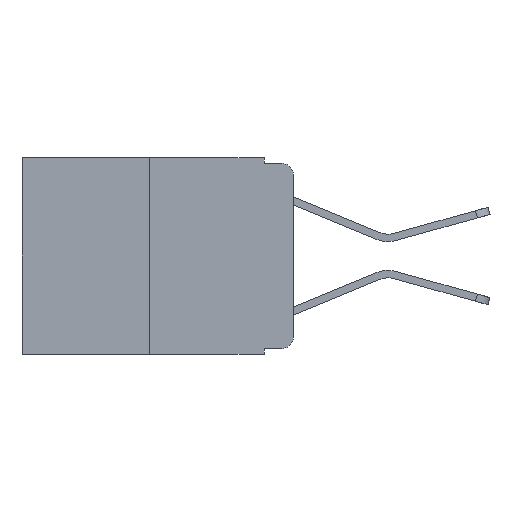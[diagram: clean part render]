
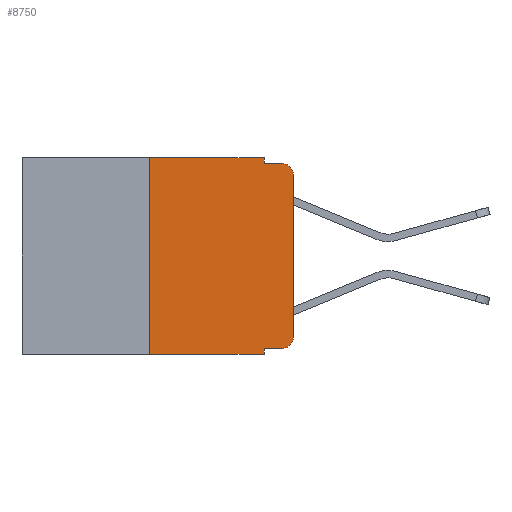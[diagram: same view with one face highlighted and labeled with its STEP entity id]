
A CAD part, left-side view. The second image highlights one B-rep face of the part: STEP entity #8750.
In plain terms, the highlighted planar face has unit normal (-1, 0, 0).
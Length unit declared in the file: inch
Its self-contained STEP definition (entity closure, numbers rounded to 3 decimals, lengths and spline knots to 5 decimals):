
#706 = CARTESIAN_POINT ( 'NONE',  ( 0., 0.473, 0. ) ) ;
#801 = CARTESIAN_POINT ( 'NONE',  ( 0., 0.051, 0. ) ) ;
#907 = ORIENTED_EDGE ( 'NONE', *, *, #7422, .T. ) ;
#1193 = CARTESIAN_POINT ( 'NONE',  ( 0., 0.02, -0.333 ) ) ;
#1472 = VERTEX_POINT ( 'NONE', #10605 ) ;
#1637 = CIRCLE ( 'NONE', #14372, 0.02 ) ;
#1759 = DIRECTION ( 'NONE',  ( 1., 0., 0. ) ) ;
#2078 = EDGE_CURVE ( 'NONE', #4910, #2132, #9257, .T. ) ;
#2132 = VERTEX_POINT ( 'NONE', #16011 ) ;
#2406 = CARTESIAN_POINT ( 'NONE',  ( 0., 0.051, -0.333 ) ) ;
#2937 = ORIENTED_EDGE ( 'NONE', *, *, #7594, .T. ) ;
#4056 = EDGE_CURVE ( 'NONE', #11079, #15684, #14596, .T. ) ;
#4217 = LINE ( 'NONE', #18147, #17213 ) ;
#4243 = DIRECTION ( 'NONE',  ( 0., -1., 0. ) ) ;
#4910 = VERTEX_POINT ( 'NONE', #20942 ) ;
#4916 = ORIENTED_EDGE ( 'NONE', *, *, #22904, .F. ) ;
#5761 = VERTEX_POINT ( 'NONE', #14639 ) ;
#6027 = LINE ( 'NONE', #6493, #14903 ) ;
#6044 = ORIENTED_EDGE ( 'NONE', *, *, #15532, .F. ) ;
#6150 = VERTEX_POINT ( 'NONE', #12118 ) ;
#6493 = CARTESIAN_POINT ( 'NONE',  ( 0., 0.051, -0.01 ) ) ;
#6593 = LINE ( 'NONE', #16574, #20034 ) ;
#6618 = CARTESIAN_POINT ( 'NONE',  ( 0., 0.02, -0.313 ) ) ;
#7011 = VECTOR ( 'NONE', #19752, 39.37008 ) ;
#7070 = CARTESIAN_POINT ( 'NONE',  ( 0., 0., 0. ) ) ;
#7422 = EDGE_CURVE ( 'NONE', #5761, #4910, #20153, .T. ) ;
#7497 = ORIENTED_EDGE ( 'NONE', *, *, #4056, .F. ) ;
#7594 = EDGE_CURVE ( 'NONE', #8365, #22496, #20950, .T. ) ;
#8307 = DIRECTION ( 'NONE',  ( 0., 0., -1. ) ) ;
#8365 = VERTEX_POINT ( 'NONE', #2406 ) ;
#8406 = AXIS2_PLACEMENT_3D ( 'NONE', #19411, #1759, #14270 ) ;
#8419 = DIRECTION ( 'NONE',  ( 0., 0., -1. ) ) ;
#8750 = ADVANCED_FACE ( 'NONE', ( #13219 ), #12527, .F. ) ;
#9007 = CARTESIAN_POINT ( 'NONE',  ( 0., 0.051, -0.343 ) ) ;
#9257 = CIRCLE ( 'NONE', #17690, 0.02 ) ;
#9309 = CARTESIAN_POINT ( 'NONE',  ( 0., 0.051, -0.333 ) ) ;
#9460 = DIRECTION ( 'NONE',  ( 0., 0., -1. ) ) ;
#9922 = VECTOR ( 'NONE', #8307, 39.37008 ) ;
#10605 = CARTESIAN_POINT ( 'NONE',  ( 0., 0.25, -0.343 ) ) ;
#10845 = LINE ( 'NONE', #11528, #14900 ) ;
#11079 = VERTEX_POINT ( 'NONE', #801 ) ;
#11185 = EDGE_CURVE ( 'NONE', #22496, #5761, #1637, .T. ) ;
#11528 = CARTESIAN_POINT ( 'NONE',  ( 0., 0.25, 0. ) ) ;
#11625 = DIRECTION ( 'NONE',  ( 0., -1., 0. ) ) ;
#11899 = DIRECTION ( 'NONE',  ( 0., -1., 0. ) ) ;
#12118 = CARTESIAN_POINT ( 'NONE',  ( 0., 0.25, 0. ) ) ;
#12527 = PLANE ( 'NONE',  #8406 ) ;
#13011 = EDGE_LOOP ( 'NONE', ( #907, #15745, #20864, #7497, #17883, #4916, #19528, #6044, #2937, #17622 ) ) ;
#13219 = FACE_OUTER_BOUND ( 'NONE', #13011, .T. ) ;
#13279 = CARTESIAN_POINT ( 'NONE',  ( 0., 0.02, -0.03 ) ) ;
#13384 = CARTESIAN_POINT ( 'NONE',  ( 0., 0.051, -0.01 ) ) ;
#14071 = EDGE_CURVE ( 'NONE', #15684, #2132, #6027, .T. ) ;
#14270 = DIRECTION ( 'NONE',  ( 0., 0., -1. ) ) ;
#14372 = AXIS2_PLACEMENT_3D ( 'NONE', #6618, #18888, #8419 ) ;
#14596 = LINE ( 'NONE', #18694, #9922 ) ;
#14639 = CARTESIAN_POINT ( 'NONE',  ( 0., 0., -0.313 ) ) ;
#14900 = VECTOR ( 'NONE', #21890, 39.37008 ) ;
#14903 = VECTOR ( 'NONE', #11899, 39.37008 ) ;
#15003 = VECTOR ( 'NONE', #19324, 39.37008 ) ;
#15532 = EDGE_CURVE ( 'NONE', #8365, #20082, #4217, .T. ) ;
#15684 = VERTEX_POINT ( 'NONE', #13384 ) ;
#15745 = ORIENTED_EDGE ( 'NONE', *, *, #2078, .T. ) ;
#16011 = CARTESIAN_POINT ( 'NONE',  ( 0., 0.02, -0.01 ) ) ;
#16263 = EDGE_CURVE ( 'NONE', #6150, #11079, #19905, .T. ) ;
#16419 = DIRECTION ( 'NONE',  ( -1., 0., 0. ) ) ;
#16574 = CARTESIAN_POINT ( 'NONE',  ( 0., 0.473, -0.343 ) ) ;
#17213 = VECTOR ( 'NONE', #9460, 39.37008 ) ;
#17622 = ORIENTED_EDGE ( 'NONE', *, *, #11185, .T. ) ;
#17690 = AXIS2_PLACEMENT_3D ( 'NONE', #13279, #16419, #18608 ) ;
#17883 = ORIENTED_EDGE ( 'NONE', *, *, #16263, .F. ) ;
#18147 = CARTESIAN_POINT ( 'NONE',  ( 0., 0.051, 0. ) ) ;
#18608 = DIRECTION ( 'NONE',  ( 0., 0., -1. ) ) ;
#18694 = CARTESIAN_POINT ( 'NONE',  ( 0., 0.051, 0. ) ) ;
#18888 = DIRECTION ( 'NONE',  ( -1., 0., 0. ) ) ;
#19038 = EDGE_CURVE ( 'NONE', #1472, #20082, #6593, .T. ) ;
#19324 = DIRECTION ( 'NONE',  ( 0., 0., 1. ) ) ;
#19370 = VECTOR ( 'NONE', #11625, 39.37008 ) ;
#19411 = CARTESIAN_POINT ( 'NONE',  ( 0., 0.473, 0. ) ) ;
#19528 = ORIENTED_EDGE ( 'NONE', *, *, #19038, .T. ) ;
#19752 = DIRECTION ( 'NONE',  ( 0., -1., 0. ) ) ;
#19905 = LINE ( 'NONE', #706, #19370 ) ;
#20034 = VECTOR ( 'NONE', #4243, 39.37008 ) ;
#20082 = VERTEX_POINT ( 'NONE', #9007 ) ;
#20153 = LINE ( 'NONE', #7070, #15003 ) ;
#20864 = ORIENTED_EDGE ( 'NONE', *, *, #14071, .F. ) ;
#20942 = CARTESIAN_POINT ( 'NONE',  ( 0., 0., -0.03 ) ) ;
#20950 = LINE ( 'NONE', #9309, #7011 ) ;
#21890 = DIRECTION ( 'NONE',  ( 0., 0., 1. ) ) ;
#22496 = VERTEX_POINT ( 'NONE', #1193 ) ;
#22904 = EDGE_CURVE ( 'NONE', #1472, #6150, #10845, .T. ) ;
